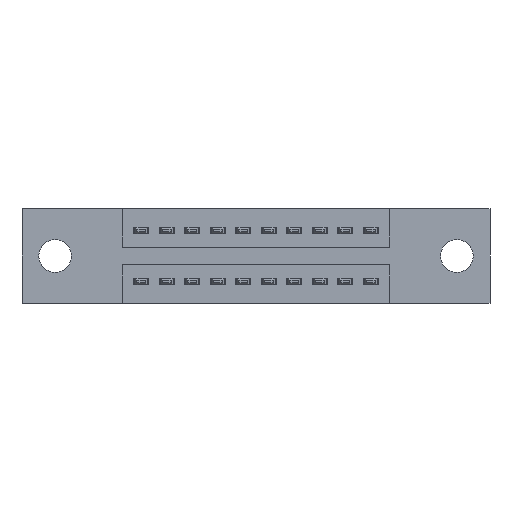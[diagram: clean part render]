
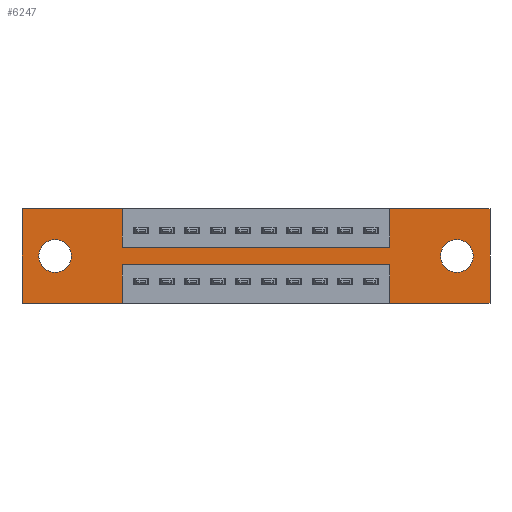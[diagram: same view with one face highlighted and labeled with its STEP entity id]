
A CAD part, front view. The second image highlights one B-rep face of the part: STEP entity #6247.
In plain terms, the highlighted planar face has unit normal (0, -1, 0).
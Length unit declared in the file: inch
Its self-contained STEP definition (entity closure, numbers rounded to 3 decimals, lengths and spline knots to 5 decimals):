
#81 = EDGE_CURVE ( 'NONE', #10294, #5811, #10903, .T. ) ;
#219 = VECTOR ( 'NONE', #7771, 39.37008 ) ;
#305 = PLANE ( 'NONE',  #7547 ) ;
#356 = CARTESIAN_POINT ( 'NONE',  ( 0., 0., -0.37 ) ) ;
#430 = DIRECTION ( 'NONE',  ( 0., 1., 0. ) ) ;
#514 = DIRECTION ( 'NONE',  ( 0., 0., -1. ) ) ;
#790 = VECTOR ( 'NONE', #4150, 39.37008 ) ;
#878 = ORIENTED_EDGE ( 'NONE', *, *, #5475, .F. ) ;
#926 = CARTESIAN_POINT ( 'NONE',  ( 0.3925, 0., -0.15 ) ) ;
#1134 = DIRECTION ( 'NONE',  ( 0., 0., -1. ) ) ;
#1142 = DIRECTION ( 'NONE',  ( 0., -1., 0. ) ) ;
#1168 = CARTESIAN_POINT ( 'NONE',  ( 0., 0., -0.37 ) ) ;
#1294 = CARTESIAN_POINT ( 'NONE',  ( 1.4425, 0., -0.22 ) ) ;
#1360 = LINE ( 'NONE', #356, #790 ) ;
#1392 = CARTESIAN_POINT ( 'NONE',  ( 1.705, 0., -0.185 ) ) ;
#1488 = EDGE_CURVE ( 'NONE', #2367, #4910, #6060, .T. ) ;
#1496 = DIRECTION ( 'NONE',  ( -1., 0., 0. ) ) ;
#1583 = CIRCLE ( 'NONE', #5221, 0.064 ) ;
#1668 = CARTESIAN_POINT ( 'NONE',  ( 0.3925, 0., -0.15 ) ) ;
#1744 = LINE ( 'NONE', #10949, #8559 ) ;
#1752 = VECTOR ( 'NONE', #1496, 39.37008 ) ;
#1855 = ORIENTED_EDGE ( 'NONE', *, *, #3429, .T. ) ;
#1865 = VERTEX_POINT ( 'NONE', #2284 ) ;
#1953 = CARTESIAN_POINT ( 'NONE',  ( 0., 0., 0. ) ) ;
#2106 = ORIENTED_EDGE ( 'NONE', *, *, #3988, .F. ) ;
#2111 = CARTESIAN_POINT ( 'NONE',  ( 1.835, 0., 0. ) ) ;
#2273 = ORIENTED_EDGE ( 'NONE', *, *, #3975, .F. ) ;
#2284 = CARTESIAN_POINT ( 'NONE',  ( 1.4425, 0., -0.37 ) ) ;
#2300 = EDGE_CURVE ( 'NONE', #3783, #11935, #2350, .T. ) ;
#2350 = LINE ( 'NONE', #1953, #2960 ) ;
#2367 = VERTEX_POINT ( 'NONE', #11493 ) ;
#2481 = CARTESIAN_POINT ( 'NONE',  ( 0.3925, 0., -0.22 ) ) ;
#2568 = ORIENTED_EDGE ( 'NONE', *, *, #1488, .T. ) ;
#2747 = DIRECTION ( 'NONE',  ( 1., 0., 0. ) ) ;
#2754 = DIRECTION ( 'NONE',  ( 0., 0., 1. ) ) ;
#2778 = ORIENTED_EDGE ( 'NONE', *, *, #6903, .F. ) ;
#2863 = ORIENTED_EDGE ( 'NONE', *, *, #7704, .T. ) ;
#2867 = DIRECTION ( 'NONE',  ( 1., 0., 0. ) ) ;
#2877 = FACE_BOUND ( 'NONE', #11405, .T. ) ;
#2878 = ORIENTED_EDGE ( 'NONE', *, *, #11787, .F. ) ;
#2960 = VECTOR ( 'NONE', #2867, 39.37008 ) ;
#3060 = DIRECTION ( 'NONE',  ( 0., 0., 1. ) ) ;
#3167 = DIRECTION ( 'NONE',  ( -1., 0., 0. ) ) ;
#3280 = LINE ( 'NONE', #926, #5913 ) ;
#3384 = VECTOR ( 'NONE', #3060, 39.37008 ) ;
#3393 = EDGE_CURVE ( 'NONE', #5550, #3783, #6904, .T. ) ;
#3429 = EDGE_CURVE ( 'NONE', #4910, #2367, #6028, .T. ) ;
#3744 = VECTOR ( 'NONE', #8187, 39.37008 ) ;
#3783 = VERTEX_POINT ( 'NONE', #10974 ) ;
#3837 = AXIS2_PLACEMENT_3D ( 'NONE', #6074, #4230, #10632 ) ;
#3910 = CARTESIAN_POINT ( 'NONE',  ( 1.835, 0., -0.37 ) ) ;
#3975 = EDGE_CURVE ( 'NONE', #8287, #10801, #7303, .T. ) ;
#3988 = EDGE_CURVE ( 'NONE', #9675, #6103, #10409, .T. ) ;
#4131 = CARTESIAN_POINT ( 'NONE',  ( 0.13, 0., -0.121 ) ) ;
#4150 = DIRECTION ( 'NONE',  ( -1., 0., 0. ) ) ;
#4161 = CARTESIAN_POINT ( 'NONE',  ( 1.4425, 0., -0.15 ) ) ;
#4230 = DIRECTION ( 'NONE',  ( 0., 1., 0. ) ) ;
#4252 = DIRECTION ( 'NONE',  ( 0., 1., 0. ) ) ;
#4307 = ORIENTED_EDGE ( 'NONE', *, *, #6864, .F. ) ;
#4345 = CIRCLE ( 'NONE', #3837, 0.064 ) ;
#4449 = ORIENTED_EDGE ( 'NONE', *, *, #3393, .F. ) ;
#4577 = ORIENTED_EDGE ( 'NONE', *, *, #10993, .T. ) ;
#4579 = CARTESIAN_POINT ( 'NONE',  ( 0., 0., -0.37 ) ) ;
#4871 = ORIENTED_EDGE ( 'NONE', *, *, #81, .F. ) ;
#4910 = VERTEX_POINT ( 'NONE', #10772 ) ;
#4965 = CARTESIAN_POINT ( 'NONE',  ( 0.3925, 0., -0.22 ) ) ;
#5063 = CARTESIAN_POINT ( 'NONE',  ( 1.705, 0., -0.185 ) ) ;
#5174 = DIRECTION ( 'NONE',  ( 0., 0., -1. ) ) ;
#5221 = AXIS2_PLACEMENT_3D ( 'NONE', #6947, #11563, #8862 ) ;
#5475 = EDGE_CURVE ( 'NONE', #7385, #1865, #11255, .T. ) ;
#5520 = VERTEX_POINT ( 'NONE', #1294 ) ;
#5524 = VECTOR ( 'NONE', #3167, 39.37008 ) ;
#5550 = VERTEX_POINT ( 'NONE', #4161 ) ;
#5700 = ORIENTED_EDGE ( 'NONE', *, *, #8838, .F. ) ;
#5747 = AXIS2_PLACEMENT_3D ( 'NONE', #5063, #430, #514 ) ;
#5811 = VERTEX_POINT ( 'NONE', #1668 ) ;
#5819 = CARTESIAN_POINT ( 'NONE',  ( 0.3925, 0., 0. ) ) ;
#5913 = VECTOR ( 'NONE', #2747, 39.37008 ) ;
#6028 = CIRCLE ( 'NONE', #5747, 0.064 ) ;
#6060 = CIRCLE ( 'NONE', #7807, 0.064 ) ;
#6074 = CARTESIAN_POINT ( 'NONE',  ( 0.13, 0., -0.185 ) ) ;
#6103 = VERTEX_POINT ( 'NONE', #7566 ) ;
#6171 = ORIENTED_EDGE ( 'NONE', *, *, #11270, .F. ) ;
#6247 = ADVANCED_FACE ( 'NONE', ( #6977, #2877, #11093 ), #305, .T. ) ;
#6271 = CARTESIAN_POINT ( 'NONE',  ( 1.835, 0., 0. ) ) ;
#6427 = CARTESIAN_POINT ( 'NONE',  ( 1.4425, 0., -0.37 ) ) ;
#6439 = EDGE_LOOP ( 'NONE', ( #2106, #8051, #2878, #878, #4307, #10032, #4449, #5700, #4871, #6171, #2273, #2778 ) ) ;
#6614 = LINE ( 'NONE', #2481, #1752 ) ;
#6748 = VECTOR ( 'NONE', #1134, 39.37008 ) ;
#6864 = EDGE_CURVE ( 'NONE', #11935, #7385, #10342, .T. ) ;
#6903 = EDGE_CURVE ( 'NONE', #6103, #8287, #1360, .T. ) ;
#6904 = LINE ( 'NONE', #11959, #7740 ) ;
#6947 = CARTESIAN_POINT ( 'NONE',  ( 0.13, 0., -0.185 ) ) ;
#6977 = FACE_BOUND ( 'NONE', #7754, .T. ) ;
#7303 = LINE ( 'NONE', #10405, #3384 ) ;
#7326 = DIRECTION ( 'NONE',  ( 0., 0., 1. ) ) ;
#7385 = VERTEX_POINT ( 'NONE', #3910 ) ;
#7547 = AXIS2_PLACEMENT_3D ( 'NONE', #8504, #1142, #10411 ) ;
#7553 = VECTOR ( 'NONE', #2754, 39.37008 ) ;
#7566 = CARTESIAN_POINT ( 'NONE',  ( 0.3925, 0., -0.37 ) ) ;
#7704 = EDGE_CURVE ( 'NONE', #8410, #7731, #4345, .T. ) ;
#7731 = VERTEX_POINT ( 'NONE', #10671 ) ;
#7740 = VECTOR ( 'NONE', #7326, 39.37008 ) ;
#7754 = EDGE_LOOP ( 'NONE', ( #2568, #1855 ) ) ;
#7771 = DIRECTION ( 'NONE',  ( 0., 0., -1. ) ) ;
#7807 = AXIS2_PLACEMENT_3D ( 'NONE', #1392, #4252, #5174 ) ;
#8051 = ORIENTED_EDGE ( 'NONE', *, *, #10387, .F. ) ;
#8187 = DIRECTION ( 'NONE',  ( 0., 0., -1. ) ) ;
#8272 = DIRECTION ( 'NONE',  ( 1., 0., 0. ) ) ;
#8287 = VERTEX_POINT ( 'NONE', #4579 ) ;
#8410 = VERTEX_POINT ( 'NONE', #4131 ) ;
#8504 = CARTESIAN_POINT ( 'NONE',  ( 0., 0., -0.37 ) ) ;
#8559 = VECTOR ( 'NONE', #8272, 39.37008 ) ;
#8838 = EDGE_CURVE ( 'NONE', #5811, #5550, #3280, .T. ) ;
#8862 = DIRECTION ( 'NONE',  ( 0., 0., 1. ) ) ;
#9410 = LINE ( 'NONE', #6427, #7553 ) ;
#9547 = CARTESIAN_POINT ( 'NONE',  ( 0.3925, 0., -0.37 ) ) ;
#9675 = VERTEX_POINT ( 'NONE', #4965 ) ;
#10032 = ORIENTED_EDGE ( 'NONE', *, *, #2300, .F. ) ;
#10294 = VERTEX_POINT ( 'NONE', #5819 ) ;
#10342 = LINE ( 'NONE', #2111, #219 ) ;
#10387 = EDGE_CURVE ( 'NONE', #5520, #9675, #6614, .T. ) ;
#10405 = CARTESIAN_POINT ( 'NONE',  ( 0., 0., 0. ) ) ;
#10409 = LINE ( 'NONE', #9547, #6748 ) ;
#10411 = DIRECTION ( 'NONE',  ( 0., 0., -1. ) ) ;
#10632 = DIRECTION ( 'NONE',  ( 0., 0., 1. ) ) ;
#10671 = CARTESIAN_POINT ( 'NONE',  ( 0.13, 0., -0.249 ) ) ;
#10772 = CARTESIAN_POINT ( 'NONE',  ( 1.705, 0., -0.249 ) ) ;
#10801 = VERTEX_POINT ( 'NONE', #11239 ) ;
#10903 = LINE ( 'NONE', #11765, #3744 ) ;
#10949 = CARTESIAN_POINT ( 'NONE',  ( 0., 0., 0. ) ) ;
#10974 = CARTESIAN_POINT ( 'NONE',  ( 1.4425, 0., 0. ) ) ;
#10993 = EDGE_CURVE ( 'NONE', #7731, #8410, #1583, .T. ) ;
#11093 = FACE_OUTER_BOUND ( 'NONE', #6439, .T. ) ;
#11239 = CARTESIAN_POINT ( 'NONE',  ( 0., 0., 0. ) ) ;
#11255 = LINE ( 'NONE', #1168, #5524 ) ;
#11270 = EDGE_CURVE ( 'NONE', #10801, #10294, #1744, .T. ) ;
#11405 = EDGE_LOOP ( 'NONE', ( #2863, #4577 ) ) ;
#11493 = CARTESIAN_POINT ( 'NONE',  ( 1.705, 0., -0.121 ) ) ;
#11563 = DIRECTION ( 'NONE',  ( 0., 1., 0. ) ) ;
#11765 = CARTESIAN_POINT ( 'NONE',  ( 0.3925, 0., 0. ) ) ;
#11787 = EDGE_CURVE ( 'NONE', #1865, #5520, #9410, .T. ) ;
#11935 = VERTEX_POINT ( 'NONE', #6271 ) ;
#11959 = CARTESIAN_POINT ( 'NONE',  ( 1.4425, 0., 0. ) ) ;
